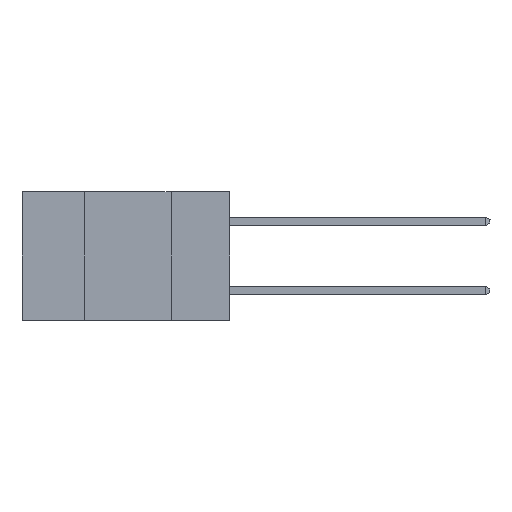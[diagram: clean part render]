
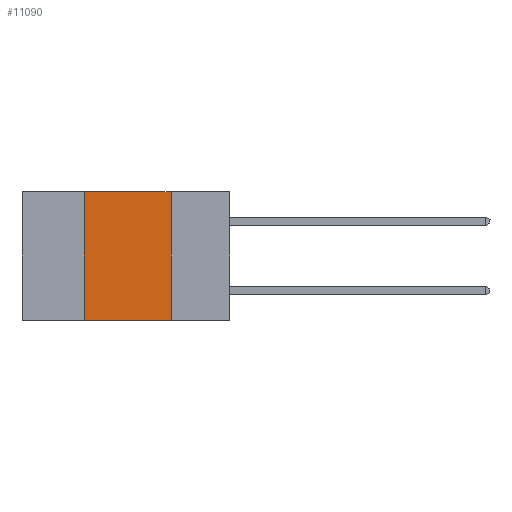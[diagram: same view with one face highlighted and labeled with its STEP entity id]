
A CAD part, left-side view. The second image highlights one B-rep face of the part: STEP entity #11090.
In plain terms, the highlighted planar face has unit normal (-1, 0, 0).
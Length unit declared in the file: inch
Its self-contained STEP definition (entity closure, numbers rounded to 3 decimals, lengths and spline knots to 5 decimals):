
#3525 = LINE ( 'NONE', #12716, #16228 ) ;
#4955 = CARTESIAN_POINT ( 'NONE',  ( 0., 0.6, -0.37 ) ) ;
#5248 = VECTOR ( 'NONE', #29175, 39.37008 ) ;
#5446 = CARTESIAN_POINT ( 'NONE',  ( 0., 0.6, 0. ) ) ;
#6906 = EDGE_CURVE ( 'NONE', #8070, #7457, #23878, .T. ) ;
#6926 = CARTESIAN_POINT ( 'NONE',  ( 0., 0.17, -0.37 ) ) ;
#7342 = VECTOR ( 'NONE', #19171, 39.37008 ) ;
#7457 = VERTEX_POINT ( 'NONE', #20606 ) ;
#7810 = DIRECTION ( 'NONE',  ( 0., 0., -1. ) ) ;
#8070 = VERTEX_POINT ( 'NONE', #8545 ) ;
#8340 = CARTESIAN_POINT ( 'NONE',  ( 0., 0.6, 0. ) ) ;
#8438 = EDGE_CURVE ( 'NONE', #9725, #8070, #11344, .T. ) ;
#8545 = CARTESIAN_POINT ( 'NONE',  ( 0., 0.42, 0. ) ) ;
#8714 = CARTESIAN_POINT ( 'NONE',  ( 0., 0.42, -0.37 ) ) ;
#9725 = VERTEX_POINT ( 'NONE', #8714 ) ;
#11090 = ADVANCED_FACE ( 'NONE', ( #29026 ), #26193, .F. ) ;
#11344 = LINE ( 'NONE', #24062, #7342 ) ;
#11988 = DIRECTION ( 'NONE',  ( 0., -1., 0. ) ) ;
#12066 = VERTEX_POINT ( 'NONE', #6926 ) ;
#12716 = CARTESIAN_POINT ( 'NONE',  ( 0., 0.17, 0. ) ) ;
#13755 = LINE ( 'NONE', #4955, #21413 ) ;
#15084 = EDGE_LOOP ( 'NONE', ( #26241, #28612, #26955, #29961 ) ) ;
#16228 = VECTOR ( 'NONE', #7810, 39.37008 ) ;
#16566 = EDGE_CURVE ( 'NONE', #7457, #12066, #3525, .T. ) ;
#17078 = DIRECTION ( 'NONE',  ( 0., 0., -1. ) ) ;
#19171 = DIRECTION ( 'NONE',  ( 0., 0., 1. ) ) ;
#20388 = AXIS2_PLACEMENT_3D ( 'NONE', #5446, #26585, #17078 ) ;
#20606 = CARTESIAN_POINT ( 'NONE',  ( 0., 0.17, 0. ) ) ;
#21406 = EDGE_CURVE ( 'NONE', #9725, #12066, #13755, .T. ) ;
#21413 = VECTOR ( 'NONE', #11988, 39.37008 ) ;
#23878 = LINE ( 'NONE', #8340, #5248 ) ;
#24062 = CARTESIAN_POINT ( 'NONE',  ( 0., 0.42, 0. ) ) ;
#26193 = PLANE ( 'NONE',  #20388 ) ;
#26241 = ORIENTED_EDGE ( 'NONE', *, *, #16566, .F. ) ;
#26585 = DIRECTION ( 'NONE',  ( 1., 0., 0. ) ) ;
#26955 = ORIENTED_EDGE ( 'NONE', *, *, #8438, .F. ) ;
#28612 = ORIENTED_EDGE ( 'NONE', *, *, #6906, .F. ) ;
#29026 = FACE_OUTER_BOUND ( 'NONE', #15084, .T. ) ;
#29175 = DIRECTION ( 'NONE',  ( 0., -1., 0. ) ) ;
#29961 = ORIENTED_EDGE ( 'NONE', *, *, #21406, .T. ) ;
